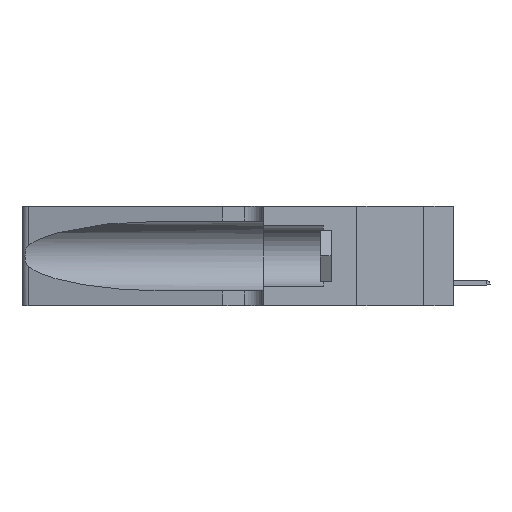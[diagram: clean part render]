
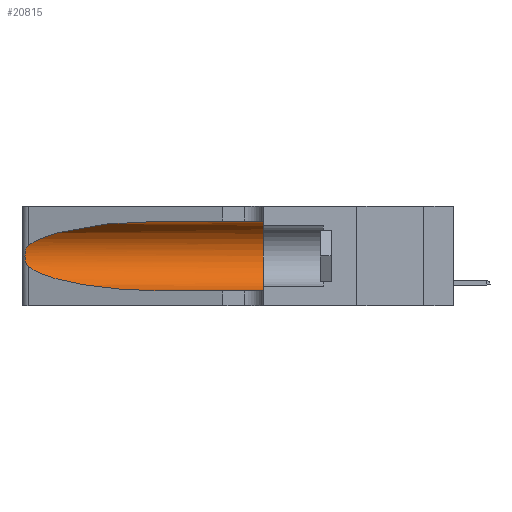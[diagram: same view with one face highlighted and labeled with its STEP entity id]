
A CAD part, left-side view. The second image highlights one B-rep face of the part: STEP entity #20815.
In plain terms, the highlighted cylindrical face has radius 3.308 mm (diameter 6.617 mm), a partial arc.
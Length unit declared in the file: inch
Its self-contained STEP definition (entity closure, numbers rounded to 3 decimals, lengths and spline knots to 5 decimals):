
#696 = CARTESIAN_POINT ( 'NONE',  ( 0.1305, 0.35, 0.05475 ) ) ;
#1390 = CARTESIAN_POINT ( 'NONE',  ( 0.26075, 1.23896, 0.178 ) ) ;
#2590 = DIRECTION ( 'NONE',  ( 0., -1., 0. ) ) ;
#2707 = CARTESIAN_POINT ( 'NONE',  ( 0.1305, 0.72297, 0.05475 ) ) ;
#2988 = EDGE_CURVE ( 'NONE', #40208, #12712, #22191, .T. ) ;
#5423 = CARTESIAN_POINT ( 'NONE',  ( 0.25639, 1.23186, 0.15144 ) ) ;
#6725 = B_SPLINE_CURVE_WITH_KNOTS ( 'NONE', 3,
 ( #37946, #23923, #41286, #9424, #38418, #8730, #41739, #1390, #30569, #34363, #23689, #5423, #38175, #23456 ),
 .UNSPECIFIED., .F., .F.,
 ( 4, 2, 2, 2, 2, 2, 4 ),
 ( 0., 0.00027, 0.00053, 0.00107, 0.0016, 0.00187, 0.00214 ),
 .UNSPECIFIED. ) ;
#8252 = VECTOR ( 'NONE', #39187, 39.37008 ) ;
#8730 = CARTESIAN_POINT ( 'NONE',  ( 0.26018, 1.23835, 0.19895 ) ) ;
#9424 = CARTESIAN_POINT ( 'NONE',  ( 0.25787, 1.23484, 0.2124 ) ) ;
#9670 = CARTESIAN_POINT ( 'NONE',  ( 0.2373, 1.15595, 0.28018 ) ) ;
#9794 = CARTESIAN_POINT ( 'NONE',  ( 0.18966, 0.96281, 0.05475 ) ) ;
#9906 = DIRECTION ( 'NONE',  ( 0., 0., -1. ) ) ;
#10423 = LINE ( 'NONE', #17321, #8252 ) ;
#10471 = CARTESIAN_POINT ( 'NONE',  ( 0.1305, 0.72297, 0.05475 ) ) ;
#11659 = DIRECTION ( 'NONE',  ( 0., 1., 0. ) ) ;
#12712 = VERTEX_POINT ( 'NONE', #37971 ) ;
#13219 = CARTESIAN_POINT ( 'NONE',  ( 0.1305, 1.61858, 0.185 ) ) ;
#13572 = VERTEX_POINT ( 'NONE', #25746 ) ;
#14195 = CIRCLE ( 'NONE', #16470, 0.13025 ) ;
#15805 = EDGE_CURVE ( 'NONE', #13572, #41609, #21636, .T. ) ;
#15861 = AXIS2_PLACEMENT_3D ( 'NONE', #13219, #2590, #9906 ) ;
#16080 = CARTESIAN_POINT ( 'NONE',  ( 0.1305, 0.72297, 0.31525 ) ) ;
#16470 = AXIS2_PLACEMENT_3D ( 'NONE', #32812, #11659, #44237 ) ;
#17321 = CARTESIAN_POINT ( 'NONE',  ( 0.1305, 1.61858, 0.05475 ) ) ;
#18473 = EDGE_CURVE ( 'NONE', #29383, #20683, #14195, .T. ) ;
#19293 = LINE ( 'NONE', #23323, #42424 ) ;
#19653 = ORIENTED_EDGE ( 'NONE', *, *, #18473, .F. ) ;
#20607 = ORIENTED_EDGE ( 'NONE', *, *, #15805, .T. ) ;
#20683 = VERTEX_POINT ( 'NONE', #696 ) ;
#20815 = ADVANCED_FACE ( 'NONE', ( #31281 ), #27258, .F. ) ;
#21636 =( BOUNDED_CURVE ( )  B_SPLINE_CURVE ( 3, ( #28062, #35441, #9794, #2707 ),
 .UNSPECIFIED., .F., .T. ) 
 B_SPLINE_CURVE_WITH_KNOTS ( ( 4, 4 ),
 ( 3.44316, 4.71239 ),
 .UNSPECIFIED. ) 
 CURVE ( )  GEOMETRIC_REPRESENTATION_ITEM ( )  RATIONAL_B_SPLINE_CURVE ( ( 1., 0.87, 0.87, 1. ) ) 
 REPRESENTATION_ITEM ( '' )  );
#22191 =( BOUNDED_CURVE ( )  B_SPLINE_CURVE ( 3, ( #16080, #27938, #9670, #41530 ),
 .UNSPECIFIED., .F., .F. ) 
 B_SPLINE_CURVE_WITH_KNOTS ( ( 4, 4 ),
 ( 1.5708, 2.84003 ),
 .UNSPECIFIED. ) 
 CURVE ( )  GEOMETRIC_REPRESENTATION_ITEM ( )  RATIONAL_B_SPLINE_CURVE ( ( 1., 0.87, 0.87, 1. ) ) 
 REPRESENTATION_ITEM ( '' )  );
#23323 = CARTESIAN_POINT ( 'NONE',  ( 0.1305, 1.61858, 0.31525 ) ) ;
#23456 = CARTESIAN_POINT ( 'NONE',  ( 0.25487, 1.22718, 0.14631 ) ) ;
#23689 = CARTESIAN_POINT ( 'NONE',  ( 0.25789, 1.23486, 0.15765 ) ) ;
#23923 = CARTESIAN_POINT ( 'NONE',  ( 0.25555, 1.22994, 0.2215 ) ) ;
#25746 = CARTESIAN_POINT ( 'NONE',  ( 0.25487, 1.22718, 0.14631 ) ) ;
#25882 = CARTESIAN_POINT ( 'NONE',  ( 0.1305, 0.35, 0.31525 ) ) ;
#27103 = DIRECTION ( 'NONE',  ( 0., -1., 0. ) ) ;
#27258 = CYLINDRICAL_SURFACE ( 'NONE', #15861, 0.13025 ) ;
#27938 = CARTESIAN_POINT ( 'NONE',  ( 0.18966, 0.96281, 0.31525 ) ) ;
#28062 = CARTESIAN_POINT ( 'NONE',  ( 0.25487, 1.22718, 0.14631 ) ) ;
#29383 = VERTEX_POINT ( 'NONE', #25882 ) ;
#29732 = CARTESIAN_POINT ( 'NONE',  ( 0.1305, 0.72297, 0.31525 ) ) ;
#29953 = EDGE_CURVE ( 'NONE', #12712, #13572, #6725, .T. ) ;
#30569 = CARTESIAN_POINT ( 'NONE',  ( 0.26017, 1.23833, 0.17102 ) ) ;
#31281 = FACE_OUTER_BOUND ( 'NONE', #46170, .T. ) ;
#32647 = ORIENTED_EDGE ( 'NONE', *, *, #37230, .F. ) ;
#32812 = CARTESIAN_POINT ( 'NONE',  ( 0.1305, 0.35, 0.185 ) ) ;
#34159 = ORIENTED_EDGE ( 'NONE', *, *, #29953, .T. ) ;
#34363 = CARTESIAN_POINT ( 'NONE',  ( 0.25856, 1.23593, 0.16098 ) ) ;
#35441 = CARTESIAN_POINT ( 'NONE',  ( 0.2373, 1.15595, 0.08982 ) ) ;
#37230 = EDGE_CURVE ( 'NONE', #40208, #29383, #19293, .T. ) ;
#37946 = CARTESIAN_POINT ( 'NONE',  ( 0.25487, 1.22718, 0.22369 ) ) ;
#37971 = CARTESIAN_POINT ( 'NONE',  ( 0.25487, 1.22718, 0.22369 ) ) ;
#38175 = CARTESIAN_POINT ( 'NONE',  ( 0.25555, 1.22993, 0.14849 ) ) ;
#38418 = CARTESIAN_POINT ( 'NONE',  ( 0.25854, 1.2359, 0.20912 ) ) ;
#38772 = ORIENTED_EDGE ( 'NONE', *, *, #2988, .T. ) ;
#39187 = DIRECTION ( 'NONE',  ( 0., -1., 0. ) ) ;
#40208 = VERTEX_POINT ( 'NONE', #29732 ) ;
#41286 = CARTESIAN_POINT ( 'NONE',  ( 0.25639, 1.23184, 0.21858 ) ) ;
#41530 = CARTESIAN_POINT ( 'NONE',  ( 0.25487, 1.22718, 0.22369 ) ) ;
#41609 = VERTEX_POINT ( 'NONE', #10471 ) ;
#41739 = CARTESIAN_POINT ( 'NONE',  ( 0.26075, 1.23896, 0.19203 ) ) ;
#41743 = ORIENTED_EDGE ( 'NONE', *, *, #43345, .T. ) ;
#42424 = VECTOR ( 'NONE', #27103, 39.37008 ) ;
#43345 = EDGE_CURVE ( 'NONE', #41609, #20683, #10423, .T. ) ;
#44237 = DIRECTION ( 'NONE',  ( 0., 0., 1. ) ) ;
#46170 = EDGE_LOOP ( 'NONE', ( #38772, #34159, #20607, #41743, #19653, #32647 ) ) ;
